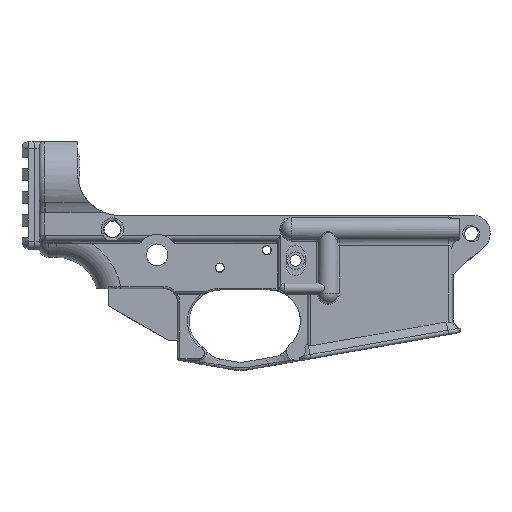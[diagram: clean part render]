
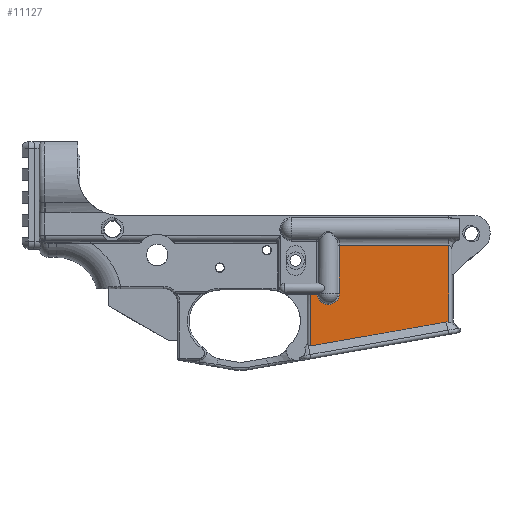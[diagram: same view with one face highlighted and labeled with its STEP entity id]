
A CAD part, left-side view. The second image highlights one B-rep face of the part: STEP entity #11127.
In plain terms, the highlighted face is planar.
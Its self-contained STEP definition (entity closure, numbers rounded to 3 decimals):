
#440=B_SPLINE_CURVE_WITH_KNOTS('',3,(#24877,#24878,#24879,#24880,#24881,
#24882),.UNSPECIFIED.,.F.,.F.,(4,2,4),(-0.114,-0.051,
0.),.UNSPECIFIED.);
#1022=PLANE('',#12272);
#1622=FACE_OUTER_BOUND('',#2282,.T.);
#2282=EDGE_LOOP('',(#10098,#10099,#10100,#10101,#10102,#10103,#10104,#10105));
#2959=LINE('',#22840,#3767);
#2960=LINE('',#22842,#3768);
#2961=LINE('',#22845,#3769);
#2962=LINE('',#22864,#3770);
#3121=LINE('',#24885,#3929);
#3122=LINE('',#24886,#3930);
#3767=VECTOR('',#14587,62.909);
#3768=VECTOR('',#14590,23.276);
#3769=VECTOR('',#14593,2.864);
#3770=VECTOR('',#14602,21.861);
#3929=VECTOR('',#15213,35.127);
#3930=VECTOR('',#15214,49.812);
#4364=CIRCLE('',#12044,5.168);
#5117=VERTEX_POINT('',#20739);
#5320=VERTEX_POINT('',#22836);
#5321=VERTEX_POINT('',#22838);
#5322=VERTEX_POINT('',#22844);
#5323=VERTEX_POINT('',#22859);
#5324=VERTEX_POINT('',#22863);
#5515=VERTEX_POINT('',#24866);
#5516=VERTEX_POINT('',#24884);
#6784=EDGE_CURVE('',#5320,#5321,#2959,.T.);
#6785=EDGE_CURVE('',#5320,#5117,#2960,.T.);
#6786=EDGE_CURVE('',#5322,#5117,#2961,.T.);
#6788=EDGE_CURVE('',#5322,#5323,#4364,.T.);
#6790=EDGE_CURVE('',#5324,#5323,#2962,.T.);
#7121=EDGE_CURVE('',#5321,#5515,#440,.T.);
#7122=EDGE_CURVE('',#5515,#5516,#3121,.T.);
#7123=EDGE_CURVE('',#5516,#5324,#3122,.T.);
#10098=ORIENTED_EDGE('',*,*,#7121,.T.);
#10099=ORIENTED_EDGE('',*,*,#7122,.T.);
#10100=ORIENTED_EDGE('',*,*,#7123,.T.);
#10101=ORIENTED_EDGE('',*,*,#6790,.T.);
#10102=ORIENTED_EDGE('',*,*,#6788,.F.);
#10103=ORIENTED_EDGE('',*,*,#6786,.T.);
#10104=ORIENTED_EDGE('',*,*,#6785,.F.);
#10105=ORIENTED_EDGE('',*,*,#6784,.T.);
#11127=ADVANCED_FACE('',(#1622),#1022,.T.);
#12044=AXIS2_PLACEMENT_3D('',#22860,#14596,#14597);
#12272=AXIS2_PLACEMENT_3D('',#24883,#15211,#15212);
#14587=DIRECTION('',(-0.985,0.174,0.));
#14590=DIRECTION('',(0.,1.,0.));
#14593=DIRECTION('',(1.,0.,0.));
#14596=DIRECTION('center_axis',(0.,0.,
-1.));
#14597=DIRECTION('ref_axis',(-1.,0.,0.));
#14602=DIRECTION('',(0.,-1.,0.));
#15211=DIRECTION('center_axis',(0.,0.,
-1.));
#15212=DIRECTION('ref_axis',(0.,-1.,0.));
#15213=DIRECTION('',(0.,1.,0.));
#15214=DIRECTION('',(1.,0.,0.));
#20739=CARTESIAN_POINT('',(471.069,131.711,-0.558));
#22836=CARTESIAN_POINT('',(471.069,108.435,-0.558));
#22838=CARTESIAN_POINT('',(409.116,119.359,-0.558));
#22840=CARTESIAN_POINT('',(471.069,108.435,-0.558));
#22842=CARTESIAN_POINT('',(471.069,108.435,-0.558));
#22844=CARTESIAN_POINT('',(468.205,131.711,-0.558));
#22845=CARTESIAN_POINT('',(468.205,131.711,-0.558));
#22859=CARTESIAN_POINT('',(457.926,132.473,-0.558));
#22860=CARTESIAN_POINT('Origin',(463.094,132.473,-0.558));
#22863=CARTESIAN_POINT('',(457.926,154.335,-0.558));
#22864=CARTESIAN_POINT('',(457.926,154.335,-0.558));
#24866=CARTESIAN_POINT('',(408.113,119.207,-0.558));
#24877=CARTESIAN_POINT('Ctrl Pts',(409.116,119.359,-0.558));
#24878=CARTESIAN_POINT('Ctrl Pts',(408.979,119.383,-0.558));
#24879=CARTESIAN_POINT('Ctrl Pts',(408.813,119.39,-0.558));
#24880=CARTESIAN_POINT('Ctrl Pts',(408.438,119.325,-0.558));
#24881=CARTESIAN_POINT('Ctrl Pts',(408.272,119.271,-0.558));
#24882=CARTESIAN_POINT('Ctrl Pts',(408.113,119.207,-0.558));
#24883=CARTESIAN_POINT('Origin',(439.591,108.159,-0.558));
#24884=CARTESIAN_POINT('',(408.113,154.335,-0.558));
#24885=CARTESIAN_POINT('',(408.113,119.207,-0.558));
#24886=CARTESIAN_POINT('',(408.113,154.335,-0.558));
